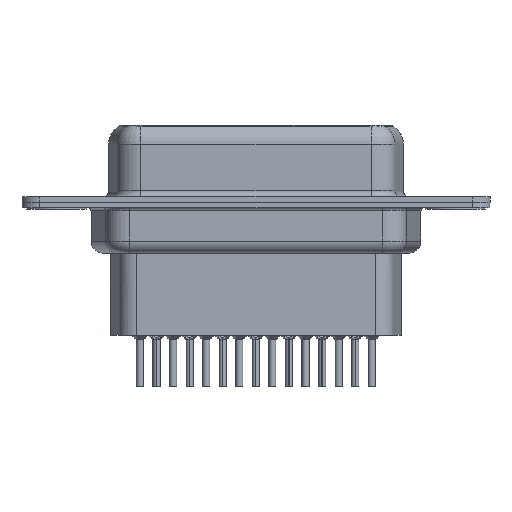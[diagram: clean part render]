
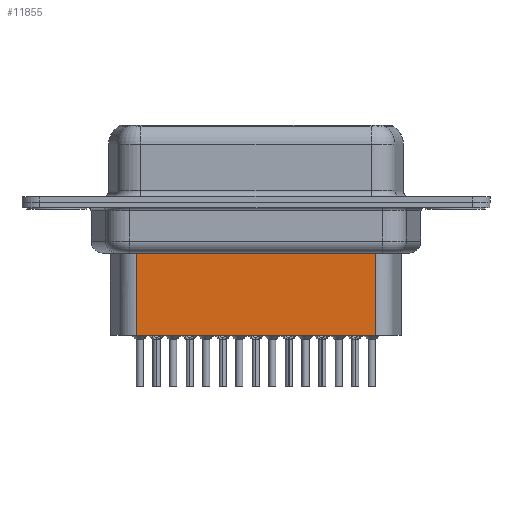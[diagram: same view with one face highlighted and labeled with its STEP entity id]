
A CAD part, front view. The second image highlights one B-rep face of the part: STEP entity #11855.
In plain terms, the highlighted planar face has unit normal (0, -1, 0).
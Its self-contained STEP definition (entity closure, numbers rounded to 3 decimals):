
#972 = DIRECTION ( 'NONE',  ( 0., 0., -1. ) ) ;
#1495 = DIRECTION ( 'NONE',  ( -1., 0., 0. ) ) ;
#1979 = DIRECTION ( 'NONE',  ( 1., 0., 0. ) ) ;
#2083 = FACE_OUTER_BOUND ( 'NONE', #4928, .T. ) ;
#2470 = CARTESIAN_POINT ( 'NONE',  ( 6.681, -3.5, -11.15 ) ) ;
#2656 = ORIENTED_EDGE ( 'NONE', *, *, #11060, .T. ) ;
#2830 = LINE ( 'NONE', #11037, #19562 ) ;
#3926 = EDGE_CURVE ( 'NONE', #15344, #15718, #4116, .T. ) ;
#4116 = LINE ( 'NONE', #16839, #7555 ) ;
#4418 = ORIENTED_EDGE ( 'NONE', *, *, #16077, .F. ) ;
#4928 = EDGE_LOOP ( 'NONE', ( #4418, #17688, #2656, #18519 ) ) ;
#5503 = VERTEX_POINT ( 'NONE', #17316 ) ;
#5572 = CARTESIAN_POINT ( 'NONE',  ( 26.619, -3.5, -11.15 ) ) ;
#6180 = LINE ( 'NONE', #2470, #11439 ) ;
#7555 = VECTOR ( 'NONE', #1495, 1000. ) ;
#10216 = VERTEX_POINT ( 'NONE', #5572 ) ;
#10977 = AXIS2_PLACEMENT_3D ( 'NONE', #17757, #17317, #1979 ) ;
#11037 = CARTESIAN_POINT ( 'NONE',  ( 6.681, -3.5, -3.1 ) ) ;
#11060 = EDGE_CURVE ( 'NONE', #15718, #5503, #2830, .T. ) ;
#11439 = VECTOR ( 'NONE', #21528, 1000. ) ;
#11855 = ADVANCED_FACE ( 'NONE', ( #2083 ), #19218, .T. ) ;
#12745 = CARTESIAN_POINT ( 'NONE',  ( 26.619, -3.5, -3.1 ) ) ;
#14291 = EDGE_CURVE ( 'NONE', #10216, #5503, #6180, .T. ) ;
#15344 = VERTEX_POINT ( 'NONE', #17300 ) ;
#15718 = VERTEX_POINT ( 'NONE', #19066 ) ;
#16077 = EDGE_CURVE ( 'NONE', #15344, #10216, #16315, .T. ) ;
#16315 = LINE ( 'NONE', #12745, #20316 ) ;
#16839 = CARTESIAN_POINT ( 'NONE',  ( 6.434, -3.5, -4.097 ) ) ;
#17300 = CARTESIAN_POINT ( 'NONE',  ( 26.619, -3.5, -4.097 ) ) ;
#17316 = CARTESIAN_POINT ( 'NONE',  ( 6.681, -3.5, -11.15 ) ) ;
#17317 = DIRECTION ( 'NONE',  ( 0., -1., 0. ) ) ;
#17688 = ORIENTED_EDGE ( 'NONE', *, *, #3926, .T. ) ;
#17757 = CARTESIAN_POINT ( 'NONE',  ( 6.681, -3.5, -3.1 ) ) ;
#18519 = ORIENTED_EDGE ( 'NONE', *, *, #14291, .F. ) ;
#19066 = CARTESIAN_POINT ( 'NONE',  ( 6.681, -3.5, -4.097 ) ) ;
#19218 = PLANE ( 'NONE',  #10977 ) ;
#19562 = VECTOR ( 'NONE', #19859, 1000. ) ;
#19859 = DIRECTION ( 'NONE',  ( 0., 0., -1. ) ) ;
#20316 = VECTOR ( 'NONE', #972, 1000. ) ;
#21528 = DIRECTION ( 'NONE',  ( -1., 0., 0. ) ) ;
